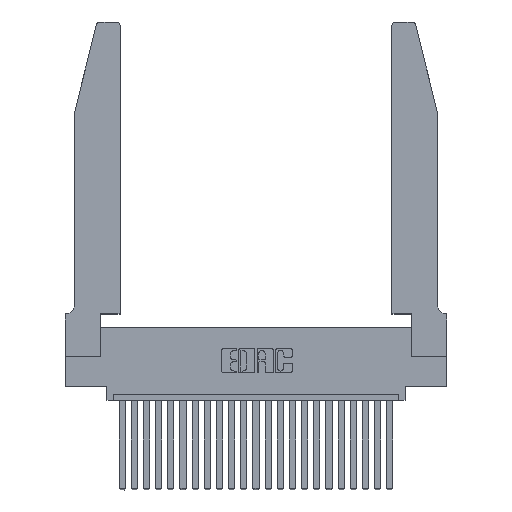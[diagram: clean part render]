
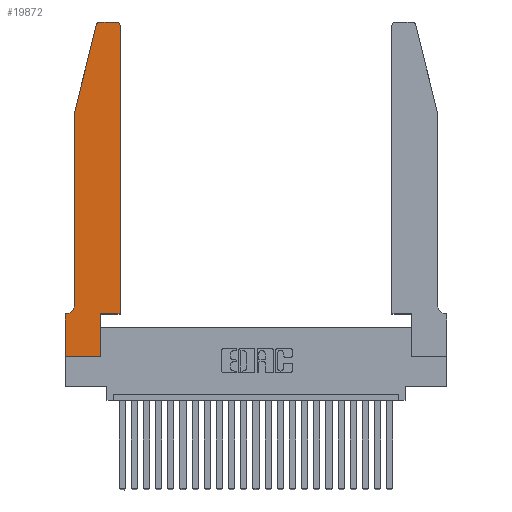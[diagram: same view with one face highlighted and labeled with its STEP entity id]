
A CAD part, top view. The second image highlights one B-rep face of the part: STEP entity #19872.
In plain terms, the highlighted planar face has unit normal (0, 0, 1).
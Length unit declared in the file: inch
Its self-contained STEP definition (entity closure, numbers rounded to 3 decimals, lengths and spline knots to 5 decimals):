
#162 = DIRECTION ( 'NONE',  ( 0., -1., 0. ) ) ;
#216 = VECTOR ( 'NONE', #3796, 39.37008 ) ;
#312 = VECTOR ( 'NONE', #19334, 39.37008 ) ;
#421 = VERTEX_POINT ( 'NONE', #10303 ) ;
#858 = CARTESIAN_POINT ( 'NONE',  ( 0., 0.35, 0.37 ) ) ;
#960 = LINE ( 'NONE', #24241, #1555 ) ;
#1094 = EDGE_CURVE ( 'NONE', #8308, #21255, #1729, .T. ) ;
#1282 = EDGE_CURVE ( 'NONE', #19422, #17188, #10928, .T. ) ;
#1555 = VECTOR ( 'NONE', #3499, 39.37008 ) ;
#1586 = EDGE_LOOP ( 'NONE', ( #6090, #16710, #20622, #22934, #13095, #20407, #4965, #4917, #11051, #20903, #11337, #8565 ) ) ;
#1729 = LINE ( 'NONE', #10777, #9458 ) ;
#1825 = CARTESIAN_POINT ( 'NONE',  ( 0.4505, 2.72, 0.37 ) ) ;
#2236 = VERTEX_POINT ( 'NONE', #858 ) ;
#2330 = CARTESIAN_POINT ( 'NONE',  ( 0.2605, 2.75, 0.37 ) ) ;
#2669 = CARTESIAN_POINT ( 'NONE',  ( 0.4205, 2.75, 0.37 ) ) ;
#2959 = VECTOR ( 'NONE', #5632, 39.37008 ) ;
#3072 = DIRECTION ( 'NONE',  ( 0., 0., 1. ) ) ;
#3099 = EDGE_CURVE ( 'NONE', #2236, #421, #6637, .T. ) ;
#3153 = PLANE ( 'NONE',  #11333 ) ;
#3499 = DIRECTION ( 'NONE',  ( -1., 0., 0. ) ) ;
#3498 = CARTESIAN_POINT ( 'NONE',  ( 0.0755, 0.42, 0.37 ) ) ;
#3796 = DIRECTION ( 'NONE',  ( 0., 1., 0. ) ) ;
#4487 = EDGE_CURVE ( 'NONE', #17188, #2236, #960, .T. ) ;
#4917 = ORIENTED_EDGE ( 'NONE', *, *, #18119, .T. ) ;
#4965 = ORIENTED_EDGE ( 'NONE', *, *, #3099, .T. ) ;
#4983 = CARTESIAN_POINT ( 'NONE',  ( 0.284, 2.75, 0.37 ) ) ;
#5385 = VECTOR ( 'NONE', #17405, 39.37008 ) ;
#5632 = DIRECTION ( 'NONE',  ( 1., 0., 0. ) ) ;
#5807 = DIRECTION ( 'NONE',  ( -1., 0., 0. ) ) ;
#6090 = ORIENTED_EDGE ( 'NONE', *, *, #17226, .T. ) ;
#6096 = CARTESIAN_POINT ( 'NONE',  ( 0.2865, 0., 0.37 ) ) ;
#6354 = DIRECTION ( 'NONE',  ( 0., 1., 0. ) ) ;
#6357 = DIRECTION ( 'NONE',  ( 0., 0., 1. ) ) ;
#6633 = VERTEX_POINT ( 'NONE', #16061 ) ;
#6637 = LINE ( 'NONE', #24417, #13176 ) ;
#7284 = CIRCLE ( 'NONE', #11125, 0.03 ) ;
#7428 = CARTESIAN_POINT ( 'NONE',  ( 0.0755, 2., 0.37 ) ) ;
#7911 = LINE ( 'NONE', #15321, #216 ) ;
#8308 = VERTEX_POINT ( 'NONE', #22402 ) ;
#8565 = ORIENTED_EDGE ( 'NONE', *, *, #14833, .T. ) ;
#9155 = CIRCLE ( 'NONE', #21920, 0.03 ) ;
#9458 = VECTOR ( 'NONE', #16344, 39.37008 ) ;
#9565 = CARTESIAN_POINT ( 'NONE',  ( 0.0055, 0.35, 0.37 ) ) ;
#9934 = CARTESIAN_POINT ( 'NONE',  ( 0.4505, 0.35, 0.37 ) ) ;
#10303 = CARTESIAN_POINT ( 'NONE',  ( 0., 0., 0.37 ) ) ;
#10682 = DIRECTION ( 'NONE',  ( 1., 0., 0. ) ) ;
#10777 = CARTESIAN_POINT ( 'NONE',  ( 0.4505, 0.35, 0.37 ) ) ;
#10849 = CARTESIAN_POINT ( 'NONE',  ( 0.0755, 2., 0.37 ) ) ;
#10928 = CIRCLE ( 'NONE', #21288, 0.07 ) ;
#11051 = ORIENTED_EDGE ( 'NONE', *, *, #15442, .T. ) ;
#11125 = AXIS2_PLACEMENT_3D ( 'NONE', #21298, #6357, #13675 ) ;
#11300 = CARTESIAN_POINT ( 'NONE',  ( 0.0055, 0.42, 0.37 ) ) ;
#11333 = AXIS2_PLACEMENT_3D ( 'NONE', #14343, #3072, #22108 ) ;
#11337 = ORIENTED_EDGE ( 'NONE', *, *, #11474, .T. ) ;
#11474 = EDGE_CURVE ( 'NONE', #21255, #12566, #7911, .T. ) ;
#11672 = CARTESIAN_POINT ( 'NONE',  ( 0., 0., 0.37 ) ) ;
#12034 = LINE ( 'NONE', #10849, #21836 ) ;
#12406 = VERTEX_POINT ( 'NONE', #2669 ) ;
#12566 = VERTEX_POINT ( 'NONE', #1825 ) ;
#12711 = VERTEX_POINT ( 'NONE', #7428 ) ;
#12719 = DIRECTION ( 'NONE',  ( -0.239, -0.971, 0. ) ) ;
#13095 = ORIENTED_EDGE ( 'NONE', *, *, #1282, .T. ) ;
#13176 = VECTOR ( 'NONE', #162, 39.37008 ) ;
#13675 = DIRECTION ( 'NONE',  ( 1., 0., 0. ) ) ;
#14343 = CARTESIAN_POINT ( 'NONE',  ( 0., 0.35, 0.37 ) ) ;
#14833 = EDGE_CURVE ( 'NONE', #12566, #12406, #7284, .T. ) ;
#14975 = VECTOR ( 'NONE', #6354, 39.37008 ) ;
#15321 = CARTESIAN_POINT ( 'NONE',  ( 0.4505, 0.35, 0.37 ) ) ;
#15442 = EDGE_CURVE ( 'NONE', #23934, #8308, #20073, .T. ) ;
#16061 = CARTESIAN_POINT ( 'NONE',  ( 0.25487, 2.72718, 0.37 ) ) ;
#16344 = DIRECTION ( 'NONE',  ( 1., 0., 0. ) ) ;
#16710 = ORIENTED_EDGE ( 'NONE', *, *, #24202, .T. ) ;
#17188 = VERTEX_POINT ( 'NONE', #9565 ) ;
#17214 = DIRECTION ( 'NONE',  ( 0., 0., -1. ) ) ;
#17226 = EDGE_CURVE ( 'NONE', #12406, #20934, #23774, .T. ) ;
#17302 = EDGE_CURVE ( 'NONE', #12711, #19422, #18801, .T. ) ;
#17405 = DIRECTION ( 'NONE',  ( -1., 0., 0. ) ) ;
#18119 = EDGE_CURVE ( 'NONE', #421, #23934, #19338, .T. ) ;
#18801 = LINE ( 'NONE', #19480, #312 ) ;
#19334 = DIRECTION ( 'NONE',  ( 0., -1., 0. ) ) ;
#19338 = LINE ( 'NONE', #11672, #2959 ) ;
#19422 = VERTEX_POINT ( 'NONE', #3498 ) ;
#19480 = CARTESIAN_POINT ( 'NONE',  ( 0.0755, 2., 0.37 ) ) ;
#19872 = ADVANCED_FACE ( 'NONE', ( #23668 ), #3153, .T. ) ;
#20073 = LINE ( 'NONE', #21293, #14975 ) ;
#20407 = ORIENTED_EDGE ( 'NONE', *, *, #4487, .T. ) ;
#20588 = EDGE_CURVE ( 'NONE', #6633, #12711, #12034, .T. ) ;
#20622 = ORIENTED_EDGE ( 'NONE', *, *, #20588, .T. ) ;
#20903 = ORIENTED_EDGE ( 'NONE', *, *, #1094, .T. ) ;
#20934 = VERTEX_POINT ( 'NONE', #4983 ) ;
#21255 = VERTEX_POINT ( 'NONE', #9934 ) ;
#21288 = AXIS2_PLACEMENT_3D ( 'NONE', #11300, #17214, #5807 ) ;
#21293 = CARTESIAN_POINT ( 'NONE',  ( 0.2865, 0.35, 0.37 ) ) ;
#21298 = CARTESIAN_POINT ( 'NONE',  ( 0.4205, 2.72, 0.37 ) ) ;
#21836 = VECTOR ( 'NONE', #12719, 39.37008 ) ;
#21920 = AXIS2_PLACEMENT_3D ( 'NONE', #22081, #22166, #10682 ) ;
#22081 = CARTESIAN_POINT ( 'NONE',  ( 0.284, 2.72, 0.37 ) ) ;
#22108 = DIRECTION ( 'NONE',  ( 1., 0., 0. ) ) ;
#22166 = DIRECTION ( 'NONE',  ( 0., 0., 1. ) ) ;
#22402 = CARTESIAN_POINT ( 'NONE',  ( 0.2865, 0.35, 0.37 ) ) ;
#22934 = ORIENTED_EDGE ( 'NONE', *, *, #17302, .T. ) ;
#23668 = FACE_OUTER_BOUND ( 'NONE', #1586, .T. ) ;
#23774 = LINE ( 'NONE', #2330, #5385 ) ;
#23934 = VERTEX_POINT ( 'NONE', #6096 ) ;
#24202 = EDGE_CURVE ( 'NONE', #20934, #6633, #9155, .T. ) ;
#24241 = CARTESIAN_POINT ( 'NONE',  ( 0.0755, 0.35, 0.37 ) ) ;
#24417 = CARTESIAN_POINT ( 'NONE',  ( 0., 0., 0.37 ) ) ;
